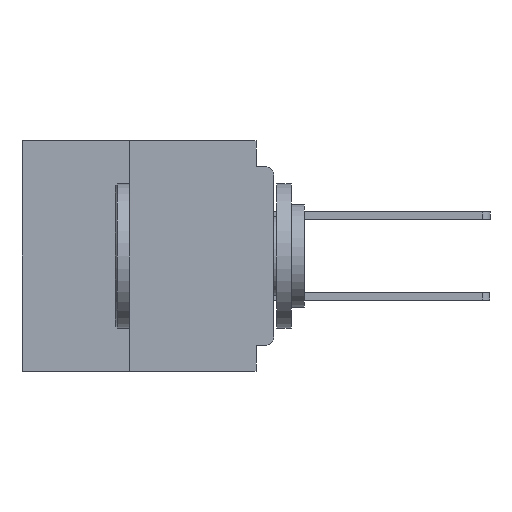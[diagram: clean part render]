
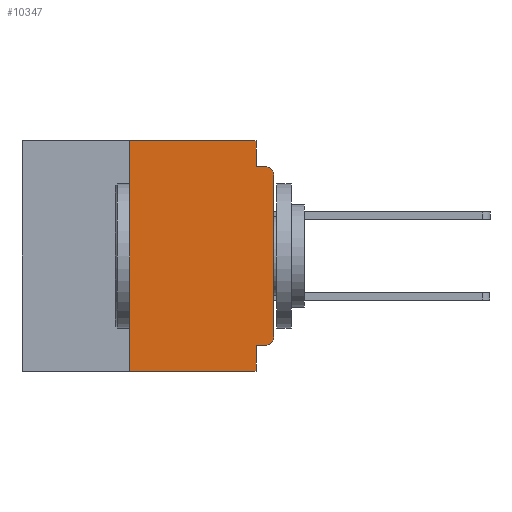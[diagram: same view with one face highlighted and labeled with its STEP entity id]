
A CAD part, left-side view. The second image highlights one B-rep face of the part: STEP entity #10347.
In plain terms, the highlighted planar face has unit normal (-1, 0, 0).
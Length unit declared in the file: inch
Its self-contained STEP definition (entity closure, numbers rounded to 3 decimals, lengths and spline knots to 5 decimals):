
#777 = VECTOR ( 'NONE', #4347, 39.37008 ) ;
#992 = DIRECTION ( 'NONE',  ( 0., 0., -1. ) ) ;
#3025 = DIRECTION ( 'NONE',  ( 0., 0., 1. ) ) ;
#3389 = LINE ( 'NONE', #24318, #13451 ) ;
#4061 = VERTEX_POINT ( 'NONE', #32573 ) ;
#4131 = VERTEX_POINT ( 'NONE', #28679 ) ;
#4347 = DIRECTION ( 'NONE',  ( 0., 0., -1. ) ) ;
#4953 = EDGE_CURVE ( 'NONE', #26619, #4131, #32104, .T. ) ;
#5105 = EDGE_CURVE ( 'NONE', #41720, #4061, #38068, .T. ) ;
#5437 = CARTESIAN_POINT ( 'NONE',  ( 0., 0.437, 0. ) ) ;
#6704 = CARTESIAN_POINT ( 'NONE',  ( 0., 0., -0.355 ) ) ;
#8040 = DIRECTION ( 'NONE',  ( 0., -1., 0. ) ) ;
#8668 = ORIENTED_EDGE ( 'NONE', *, *, #24098, .F. ) ;
#9653 = EDGE_CURVE ( 'NONE', #24802, #12071, #23735, .T. ) ;
#10347 = ADVANCED_FACE ( 'NONE', ( #21684 ), #14047, .F. ) ;
#10390 = LINE ( 'NONE', #17013, #23092 ) ;
#10639 = CIRCLE ( 'NONE', #36625, 0.015 ) ;
#10707 = EDGE_CURVE ( 'NONE', #23220, #4131, #14274, .T. ) ;
#12071 = VERTEX_POINT ( 'NONE', #21153 ) ;
#12424 = CARTESIAN_POINT ( 'NONE',  ( 0., 0., -0.06 ) ) ;
#13451 = VECTOR ( 'NONE', #3025, 39.37008 ) ;
#13928 = CARTESIAN_POINT ( 'NONE',  ( 0., 0.031, 0. ) ) ;
#13993 = DIRECTION ( 'NONE',  ( 0., -1., 0. ) ) ;
#14047 = PLANE ( 'NONE',  #32580 ) ;
#14274 = LINE ( 'NONE', #33539, #48185 ) ;
#14986 = ORIENTED_EDGE ( 'NONE', *, *, #5105, .T. ) ;
#16941 = CARTESIAN_POINT ( 'NONE',  ( 0., 0.015, -0.06 ) ) ;
#17013 = CARTESIAN_POINT ( 'NONE',  ( 0., 0., 0. ) ) ;
#17290 = CARTESIAN_POINT ( 'NONE',  ( 0., 0.031, -0.355 ) ) ;
#18334 = DIRECTION ( 'NONE',  ( 1., 0., 0. ) ) ;
#19509 = ORIENTED_EDGE ( 'NONE', *, *, #40590, .F. ) ;
#21153 = CARTESIAN_POINT ( 'NONE',  ( 0., 0.031, -0.045 ) ) ;
#21247 = DIRECTION ( 'NONE',  ( 0., 0., -1. ) ) ;
#21313 = ORIENTED_EDGE ( 'NONE', *, *, #10707, .T. ) ;
#21684 = FACE_OUTER_BOUND ( 'NONE', #51888, .T. ) ;
#22857 = ORIENTED_EDGE ( 'NONE', *, *, #9653, .F. ) ;
#23035 = ORIENTED_EDGE ( 'NONE', *, *, #31228, .T. ) ;
#23092 = VECTOR ( 'NONE', #42466, 39.37008 ) ;
#23186 = AXIS2_PLACEMENT_3D ( 'NONE', #52008, #26542, #992 ) ;
#23220 = VERTEX_POINT ( 'NONE', #29892 ) ;
#23735 = LINE ( 'NONE', #52948, #33693 ) ;
#24098 = EDGE_CURVE ( 'NONE', #41720, #26619, #52958, .T. ) ;
#24318 = CARTESIAN_POINT ( 'NONE',  ( 0., 0.25, -0.4 ) ) ;
#24754 = ORIENTED_EDGE ( 'NONE', *, *, #29466, .F. ) ;
#24802 = VERTEX_POINT ( 'NONE', #13928 ) ;
#26309 = CARTESIAN_POINT ( 'NONE',  ( 0., 0.015, -0.045 ) ) ;
#26542 = DIRECTION ( 'NONE',  ( -1., 0., 0. ) ) ;
#26619 = VERTEX_POINT ( 'NONE', #17290 ) ;
#26748 = CARTESIAN_POINT ( 'NONE',  ( 0., 0.015, -0.355 ) ) ;
#28128 = DIRECTION ( 'NONE',  ( 0., 1., 0. ) ) ;
#28580 = ORIENTED_EDGE ( 'NONE', *, *, #4953, .F. ) ;
#28648 = VECTOR ( 'NONE', #29275, 39.37008 ) ;
#28679 = CARTESIAN_POINT ( 'NONE',  ( 0., 0.031, -0.4 ) ) ;
#28861 = ORIENTED_EDGE ( 'NONE', *, *, #33531, .F. ) ;
#29275 = DIRECTION ( 'NONE',  ( 0., -1., 0. ) ) ;
#29466 = EDGE_CURVE ( 'NONE', #12071, #45436, #33238, .T. ) ;
#29892 = CARTESIAN_POINT ( 'NONE',  ( 0., 0.25, -0.4 ) ) ;
#29909 = CARTESIAN_POINT ( 'NONE',  ( 0., 0.031, -0.4 ) ) ;
#31228 = EDGE_CURVE ( 'NONE', #4061, #32341, #10390, .T. ) ;
#31673 = VERTEX_POINT ( 'NONE', #45574 ) ;
#31774 = DIRECTION ( 'NONE',  ( 0., 0., -1. ) ) ;
#32104 = LINE ( 'NONE', #29909, #777 ) ;
#32341 = VERTEX_POINT ( 'NONE', #12424 ) ;
#32573 = CARTESIAN_POINT ( 'NONE',  ( 0., 0., -0.34 ) ) ;
#32580 = AXIS2_PLACEMENT_3D ( 'NONE', #5437, #18334, #48049 ) ;
#33238 = LINE ( 'NONE', #39446, #44532 ) ;
#33531 = EDGE_CURVE ( 'NONE', #23220, #31673, #3389, .T. ) ;
#33539 = CARTESIAN_POINT ( 'NONE',  ( 0., 0.437, -0.4 ) ) ;
#33693 = VECTOR ( 'NONE', #31774, 39.37008 ) ;
#36625 = AXIS2_PLACEMENT_3D ( 'NONE', #16941, #46649, #21247 ) ;
#38068 = CIRCLE ( 'NONE', #23186, 0.015 ) ;
#39359 = EDGE_CURVE ( 'NONE', #32341, #45436, #10639, .T. ) ;
#39446 = CARTESIAN_POINT ( 'NONE',  ( 0., 0., -0.045 ) ) ;
#40308 = VECTOR ( 'NONE', #28128, 39.37008 ) ;
#40590 = EDGE_CURVE ( 'NONE', #31673, #24802, #49927, .T. ) ;
#41720 = VERTEX_POINT ( 'NONE', #26748 ) ;
#42445 = ORIENTED_EDGE ( 'NONE', *, *, #39359, .T. ) ;
#42466 = DIRECTION ( 'NONE',  ( 0., 0., 1. ) ) ;
#44532 = VECTOR ( 'NONE', #13993, 39.37008 ) ;
#45436 = VERTEX_POINT ( 'NONE', #26309 ) ;
#45574 = CARTESIAN_POINT ( 'NONE',  ( 0., 0.25, 0. ) ) ;
#46649 = DIRECTION ( 'NONE',  ( -1., 0., 0. ) ) ;
#48049 = DIRECTION ( 'NONE',  ( 0., 0., -1. ) ) ;
#48185 = VECTOR ( 'NONE', #8040, 39.37008 ) ;
#49927 = LINE ( 'NONE', #54690, #28648 ) ;
#51888 = EDGE_LOOP ( 'NONE', ( #23035, #42445, #24754, #22857, #19509, #28861, #21313, #28580, #8668, #14986 ) ) ;
#52008 = CARTESIAN_POINT ( 'NONE',  ( 0., 0.015, -0.34 ) ) ;
#52948 = CARTESIAN_POINT ( 'NONE',  ( 0., 0.031, 0. ) ) ;
#52958 = LINE ( 'NONE', #6704, #40308 ) ;
#54690 = CARTESIAN_POINT ( 'NONE',  ( 0., 0.437, 0. ) ) ;
